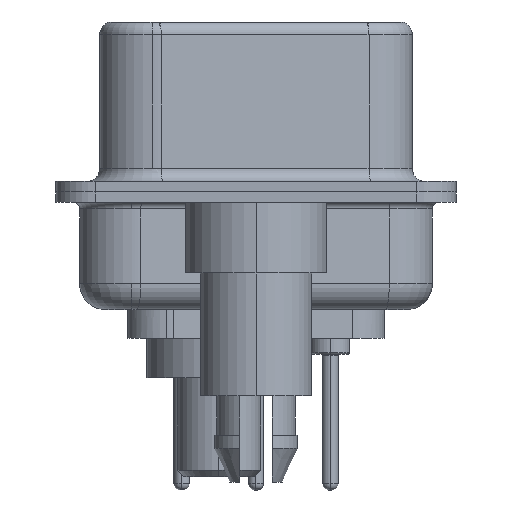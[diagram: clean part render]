
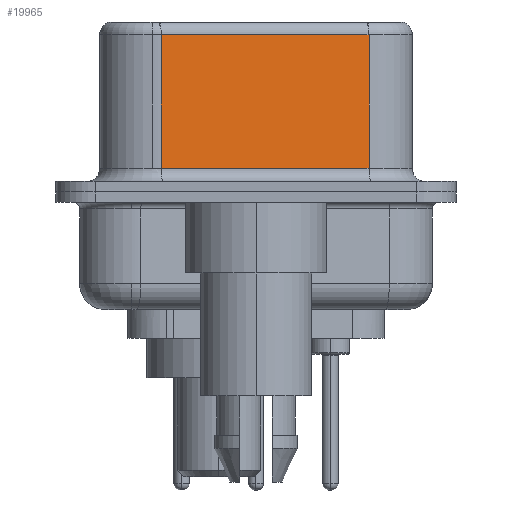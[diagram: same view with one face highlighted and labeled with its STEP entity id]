
A CAD part, left-side view. The second image highlights one B-rep face of the part: STEP entity #19965.
In plain terms, the highlighted planar face has unit normal (-0.985, -0.174, 0).
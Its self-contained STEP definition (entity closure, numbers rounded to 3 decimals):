
#1103 = VERTEX_POINT ( 'NONE', #11666 ) ;
#1212 = DIRECTION ( 'NONE',  ( 0.174, -0.985, 0. ) ) ;
#1866 = EDGE_CURVE ( 'NONE', #25168, #2353, #25338, .T. ) ;
#2353 = VERTEX_POINT ( 'NONE', #12772 ) ;
#2507 = PLANE ( 'NONE',  #6313 ) ;
#2543 = EDGE_CURVE ( 'NONE', #1103, #14262, #12207, .T. ) ;
#3519 = ORIENTED_EDGE ( 'NONE', *, *, #2543, .T. ) ;
#4308 = VECTOR ( 'NONE', #10561, 1000. ) ;
#4435 = EDGE_CURVE ( 'NONE', #25168, #14262, #13742, .T. ) ;
#4615 = DIRECTION ( 'NONE',  ( 0.985, 0.174, 0. ) ) ;
#5431 = CARTESIAN_POINT ( 'NONE',  ( 5.132, -4.322, 6.02 ) ) ;
#6313 = AXIS2_PLACEMENT_3D ( 'NONE', #15080, #4615, #19318 ) ;
#8203 = CARTESIAN_POINT ( 'NONE',  ( 5.132, -4.322, 0.9 ) ) ;
#10561 = DIRECTION ( 'NONE',  ( -0.174, 0.985, 0. ) ) ;
#10701 = ORIENTED_EDGE ( 'NONE', *, *, #4435, .F. ) ;
#10888 = CARTESIAN_POINT ( 'NONE',  ( 5.132, -4.322, 6.02 ) ) ;
#11353 = DIRECTION ( 'NONE',  ( 0., 0., -1. ) ) ;
#11666 = CARTESIAN_POINT ( 'NONE',  ( 3.73, 3.628, 0.9 ) ) ;
#12207 = LINE ( 'NONE', #13856, #18386 ) ;
#12293 = EDGE_LOOP ( 'NONE', ( #10701, #22770, #26635, #3519 ) ) ;
#12772 = CARTESIAN_POINT ( 'NONE',  ( 3.73, 3.628, 6.02 ) ) ;
#13643 = VECTOR ( 'NONE', #11353, 1000. ) ;
#13742 = LINE ( 'NONE', #18661, #24233 ) ;
#13856 = CARTESIAN_POINT ( 'NONE',  ( 5.132, -4.322, 0.9 ) ) ;
#14262 = VERTEX_POINT ( 'NONE', #8203 ) ;
#15080 = CARTESIAN_POINT ( 'NONE',  ( 5.132, -4.322, 6.52 ) ) ;
#18386 = VECTOR ( 'NONE', #1212, 1000. ) ;
#18661 = CARTESIAN_POINT ( 'NONE',  ( 5.132, -4.322, 6.52 ) ) ;
#19318 = DIRECTION ( 'NONE',  ( -0.174, 0.985, 0. ) ) ;
#19368 = DIRECTION ( 'NONE',  ( 0., 0., -1. ) ) ;
#19965 = ADVANCED_FACE ( 'NONE', ( #22521 ), #2507, .F. ) ;
#20108 = EDGE_CURVE ( 'NONE', #2353, #1103, #24785, .T. ) ;
#22521 = FACE_OUTER_BOUND ( 'NONE', #12293, .T. ) ;
#22770 = ORIENTED_EDGE ( 'NONE', *, *, #1866, .T. ) ;
#23899 = CARTESIAN_POINT ( 'NONE',  ( 3.73, 3.628, 6.52 ) ) ;
#24233 = VECTOR ( 'NONE', #19368, 1000. ) ;
#24785 = LINE ( 'NONE', #23899, #13643 ) ;
#25168 = VERTEX_POINT ( 'NONE', #10888 ) ;
#25338 = LINE ( 'NONE', #5431, #4308 ) ;
#26635 = ORIENTED_EDGE ( 'NONE', *, *, #20108, .T. ) ;
